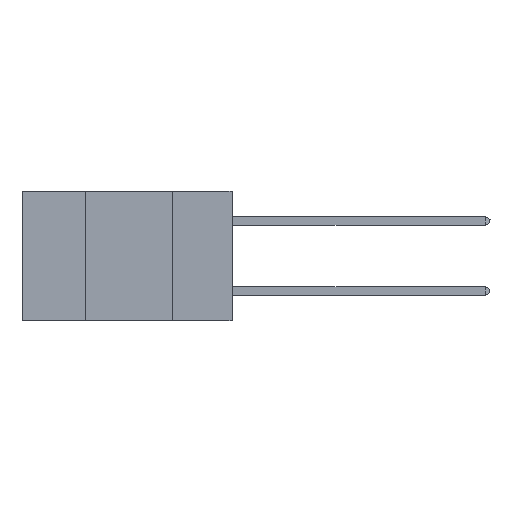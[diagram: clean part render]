
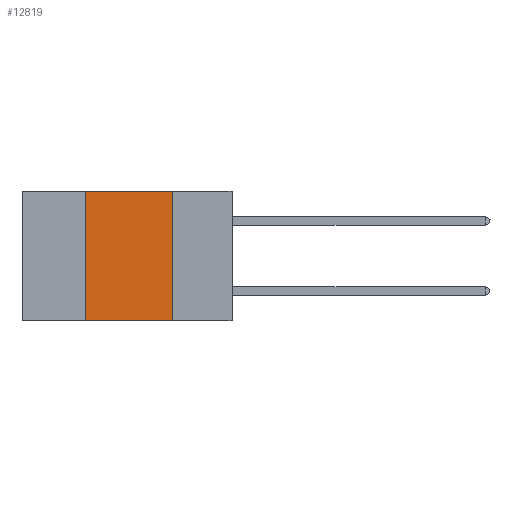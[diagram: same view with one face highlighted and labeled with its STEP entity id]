
A CAD part, left-side view. The second image highlights one B-rep face of the part: STEP entity #12819.
In plain terms, the highlighted planar face has unit normal (-1, 0, 0).
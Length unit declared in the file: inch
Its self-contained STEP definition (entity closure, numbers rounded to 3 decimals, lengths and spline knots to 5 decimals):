
#238 = ORIENTED_EDGE ( 'NONE', *, *, #13358, .F. ) ;
#1118 = VERTEX_POINT ( 'NONE', #6510 ) ;
#1129 = DIRECTION ( 'NONE',  ( 0., -1., 0. ) ) ;
#1167 = VERTEX_POINT ( 'NONE', #13569 ) ;
#1660 = FACE_OUTER_BOUND ( 'NONE', #2241, .T. ) ;
#1701 = DIRECTION ( 'NONE',  ( 0., 0., -1. ) ) ;
#2241 = EDGE_LOOP ( 'NONE', ( #10280, #238, #6472, #9211 ) ) ;
#2891 = DIRECTION ( 'NONE',  ( 0., 0., -1. ) ) ;
#4093 = CARTESIAN_POINT ( 'NONE',  ( 0., 0.42, 0. ) ) ;
#4253 = VERTEX_POINT ( 'NONE', #11818 ) ;
#4366 = VECTOR ( 'NONE', #9514, 39.37008 ) ;
#4827 = CARTESIAN_POINT ( 'NONE',  ( 0., 0.42, 0. ) ) ;
#5488 = PLANE ( 'NONE',  #12489 ) ;
#6046 = VECTOR ( 'NONE', #1701, 39.37008 ) ;
#6133 = LINE ( 'NONE', #4827, #4366 ) ;
#6472 = ORIENTED_EDGE ( 'NONE', *, *, #13671, .F. ) ;
#6510 = CARTESIAN_POINT ( 'NONE',  ( 0., 0.42, -0.37 ) ) ;
#7367 = CARTESIAN_POINT ( 'NONE',  ( 0., 0.17, 0. ) ) ;
#7446 = LINE ( 'NONE', #7367, #6046 ) ;
#7494 = EDGE_CURVE ( 'NONE', #1167, #4253, #7446, .T. ) ;
#8012 = LINE ( 'NONE', #11609, #11039 ) ;
#8806 = DIRECTION ( 'NONE',  ( 1., 0., 0. ) ) ;
#9075 = VECTOR ( 'NONE', #12446, 39.37008 ) ;
#9211 = ORIENTED_EDGE ( 'NONE', *, *, #12991, .T. ) ;
#9514 = DIRECTION ( 'NONE',  ( 0., 0., 1. ) ) ;
#10280 = ORIENTED_EDGE ( 'NONE', *, *, #7494, .F. ) ;
#11039 = VECTOR ( 'NONE', #1129, 39.37008 ) ;
#11236 = LINE ( 'NONE', #13525, #9075 ) ;
#11609 = CARTESIAN_POINT ( 'NONE',  ( 0., 0.6, -0.37 ) ) ;
#11818 = CARTESIAN_POINT ( 'NONE',  ( 0., 0.17, -0.37 ) ) ;
#12446 = DIRECTION ( 'NONE',  ( 0., -1., 0. ) ) ;
#12489 = AXIS2_PLACEMENT_3D ( 'NONE', #14623, #8806, #2891 ) ;
#12819 = ADVANCED_FACE ( 'NONE', ( #1660 ), #5488, .F. ) ;
#12991 = EDGE_CURVE ( 'NONE', #1118, #4253, #8012, .T. ) ;
#13311 = VERTEX_POINT ( 'NONE', #4093 ) ;
#13358 = EDGE_CURVE ( 'NONE', #13311, #1167, #11236, .T. ) ;
#13525 = CARTESIAN_POINT ( 'NONE',  ( 0., 0.6, 0. ) ) ;
#13569 = CARTESIAN_POINT ( 'NONE',  ( 0., 0.17, 0. ) ) ;
#13671 = EDGE_CURVE ( 'NONE', #1118, #13311, #6133, .T. ) ;
#14623 = CARTESIAN_POINT ( 'NONE',  ( 0., 0.6, 0. ) ) ;
